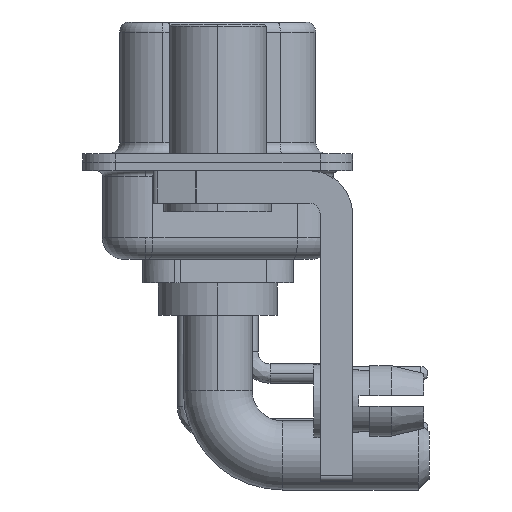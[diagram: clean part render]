
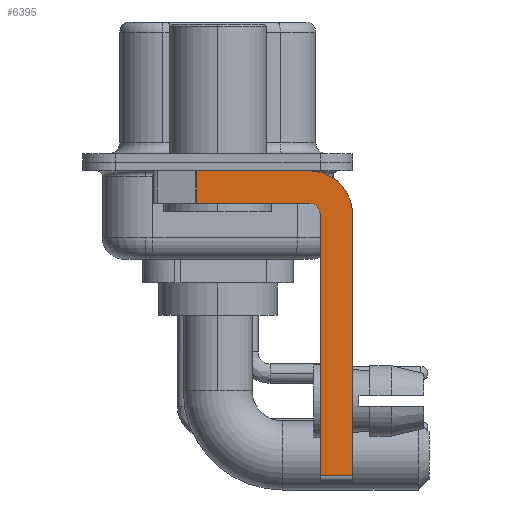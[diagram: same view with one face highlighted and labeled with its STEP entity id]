
A CAD part, left-side view. The second image highlights one B-rep face of the part: STEP entity #6395.
In plain terms, the highlighted planar face has unit normal (-1, 0, 0).
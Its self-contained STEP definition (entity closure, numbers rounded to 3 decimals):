
#11 = CARTESIAN_POINT ( 'NONE',  ( -2.9, -4.25, -1.9 ) ) ;
#811 = VECTOR ( 'NONE', #27177, 1000. ) ;
#884 = DIRECTION ( 'NONE',  ( 1., 0., 0. ) ) ;
#2280 = CARTESIAN_POINT ( 'NONE',  ( -2.9, 3., -0.4 ) ) ;
#2656 = AXIS2_PLACEMENT_3D ( 'NONE', #8389, #12830, #21548 ) ;
#2755 = DIRECTION ( 'NONE',  ( 0., 0., -1. ) ) ;
#2892 = FACE_OUTER_BOUND ( 'NONE', #5828, .T. ) ;
#2894 = LINE ( 'NONE', #15919, #17748 ) ;
#3250 = VERTEX_POINT ( 'NONE', #6102 ) ;
#3648 = EDGE_CURVE ( 'NONE', #12789, #3250, #23765, .T. ) ;
#3815 = EDGE_CURVE ( 'NONE', #12789, #19255, #9576, .T. ) ;
#3823 = VECTOR ( 'NONE', #15043, 1000. ) ;
#4654 = ORIENTED_EDGE ( 'NONE', *, *, #18757, .F. ) ;
#4816 = CARTESIAN_POINT ( 'NONE',  ( -2.9, -6.25, -2.4 ) ) ;
#5017 = CIRCLE ( 'NONE', #2656, 0.5 ) ;
#5139 = DIRECTION ( 'NONE',  ( 0., 0., -1. ) ) ;
#5202 = AXIS2_PLACEMENT_3D ( 'NONE', #22202, #9625, #15918 ) ;
#5828 = EDGE_LOOP ( 'NONE', ( #8959, #26234, #4654, #13330, #20855, #8437, #12861, #24768 ) ) ;
#5838 = LINE ( 'NONE', #20560, #7431 ) ;
#6102 = CARTESIAN_POINT ( 'NONE',  ( -2.9, -4.25, -0.4 ) ) ;
#6395 = ADVANCED_FACE ( 'NONE', ( #2892 ), #9056, .F. ) ;
#7431 = VECTOR ( 'NONE', #10130, 1000. ) ;
#8291 = EDGE_CURVE ( 'NONE', #27534, #24488, #14020, .T. ) ;
#8389 = CARTESIAN_POINT ( 'NONE',  ( -2.9, -4.25, -2.4 ) ) ;
#8437 = ORIENTED_EDGE ( 'NONE', *, *, #23004, .T. ) ;
#8959 = ORIENTED_EDGE ( 'NONE', *, *, #3648, .F. ) ;
#9056 = PLANE ( 'NONE',  #5202 ) ;
#9570 = AXIS2_PLACEMENT_3D ( 'NONE', #20068, #884, #26928 ) ;
#9576 = LINE ( 'NONE', #24597, #17979 ) ;
#9625 = DIRECTION ( 'NONE',  ( 1., 0., 0. ) ) ;
#10130 = DIRECTION ( 'NONE',  ( 0., 1., 0. ) ) ;
#10230 = EDGE_CURVE ( 'NONE', #24488, #19471, #5017, .T. ) ;
#10606 = CARTESIAN_POINT ( 'NONE',  ( -2.9, -4.75, -2.4 ) ) ;
#11275 = VERTEX_POINT ( 'NONE', #15492 ) ;
#11336 = EDGE_CURVE ( 'NONE', #3250, #26641, #11852, .T. ) ;
#11852 = CIRCLE ( 'NONE', #9570, 2. ) ;
#12756 = LINE ( 'NONE', #19602, #23995 ) ;
#12789 = VERTEX_POINT ( 'NONE', #24213 ) ;
#12830 = DIRECTION ( 'NONE',  ( -1., 0., 0. ) ) ;
#12861 = ORIENTED_EDGE ( 'NONE', *, *, #28101, .F. ) ;
#13252 = CARTESIAN_POINT ( 'NONE',  ( -2.9, -4.75, -14.55 ) ) ;
#13330 = ORIENTED_EDGE ( 'NONE', *, *, #10230, .F. ) ;
#14020 = LINE ( 'NONE', #22750, #811 ) ;
#15043 = DIRECTION ( 'NONE',  ( 0., -1., 0. ) ) ;
#15492 = CARTESIAN_POINT ( 'NONE',  ( -2.9, -6.25, -14.55 ) ) ;
#15918 = DIRECTION ( 'NONE',  ( 0., 0., -1. ) ) ;
#15919 = CARTESIAN_POINT ( 'NONE',  ( -2.9, -6.25, -2.4 ) ) ;
#17748 = VECTOR ( 'NONE', #2755, 1000. ) ;
#17979 = VECTOR ( 'NONE', #5139, 1000. ) ;
#18757 = EDGE_CURVE ( 'NONE', #19471, #19255, #5838, .T. ) ;
#19255 = VERTEX_POINT ( 'NONE', #27635 ) ;
#19471 = VERTEX_POINT ( 'NONE', #11 ) ;
#19602 = CARTESIAN_POINT ( 'NONE',  ( -2.9, -4.25, -14.55 ) ) ;
#19874 = DIRECTION ( 'NONE',  ( 0., -1., 0. ) ) ;
#20068 = CARTESIAN_POINT ( 'NONE',  ( -2.9, -4.25, -2.4 ) ) ;
#20560 = CARTESIAN_POINT ( 'NONE',  ( -2.9, -4.25, -1.9 ) ) ;
#20855 = ORIENTED_EDGE ( 'NONE', *, *, #8291, .F. ) ;
#21548 = DIRECTION ( 'NONE',  ( 0., 0., 1. ) ) ;
#22202 = CARTESIAN_POINT ( 'NONE',  ( -2.9, -4.25, -2.4 ) ) ;
#22750 = CARTESIAN_POINT ( 'NONE',  ( -2.9, -4.75, -14.8 ) ) ;
#23004 = EDGE_CURVE ( 'NONE', #27534, #11275, #12756, .T. ) ;
#23765 = LINE ( 'NONE', #2280, #3823 ) ;
#23995 = VECTOR ( 'NONE', #19874, 1000. ) ;
#24213 = CARTESIAN_POINT ( 'NONE',  ( -2.9, 0.978, -0.4 ) ) ;
#24488 = VERTEX_POINT ( 'NONE', #10606 ) ;
#24597 = CARTESIAN_POINT ( 'NONE',  ( -2.9, 0.978, -1.9 ) ) ;
#24768 = ORIENTED_EDGE ( 'NONE', *, *, #11336, .F. ) ;
#26234 = ORIENTED_EDGE ( 'NONE', *, *, #3815, .T. ) ;
#26641 = VERTEX_POINT ( 'NONE', #4816 ) ;
#26928 = DIRECTION ( 'NONE',  ( 0., 0., -1. ) ) ;
#27177 = DIRECTION ( 'NONE',  ( 0., 0., 1. ) ) ;
#27534 = VERTEX_POINT ( 'NONE', #13252 ) ;
#27635 = CARTESIAN_POINT ( 'NONE',  ( -2.9, 0.978, -1.9 ) ) ;
#28101 = EDGE_CURVE ( 'NONE', #26641, #11275, #2894, .T. ) ;
